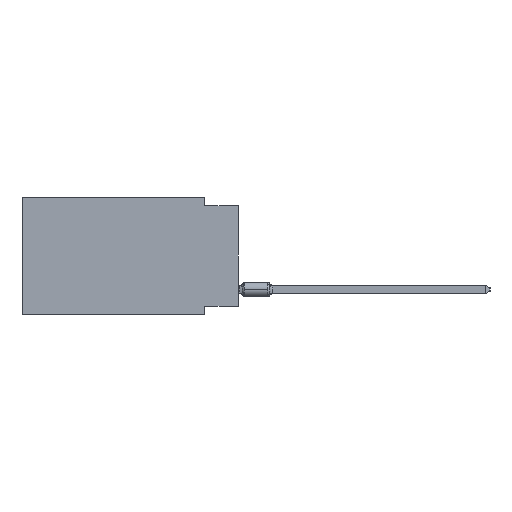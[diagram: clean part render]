
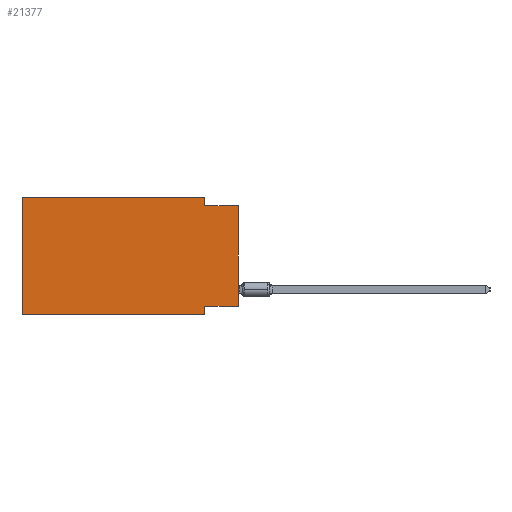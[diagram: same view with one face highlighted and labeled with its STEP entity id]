
A CAD part, left-side view. The second image highlights one B-rep face of the part: STEP entity #21377.
In plain terms, the highlighted planar face has unit normal (-1, 0, 0).
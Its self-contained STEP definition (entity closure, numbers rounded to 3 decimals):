
#441 = CARTESIAN_POINT ( 'NONE',  ( 0., 16.383, 0. ) ) ;
#513 = VECTOR ( 'NONE', #53998, 1000. ) ;
#1346 = DIRECTION ( 'NONE',  ( 0., 0., 1. ) ) ;
#3556 = VERTEX_POINT ( 'NONE', #6404 ) ;
#6296 = CARTESIAN_POINT ( 'NONE',  ( 0., 0., -0.635 ) ) ;
#6312 = CARTESIAN_POINT ( 'NONE',  ( 0., 0., -8.255 ) ) ;
#6404 = CARTESIAN_POINT ( 'NONE',  ( 0., 2.54, -8.89 ) ) ;
#7161 = VERTEX_POINT ( 'NONE', #33942 ) ;
#10131 = VECTOR ( 'NONE', #59134, 1000. ) ;
#10188 = VERTEX_POINT ( 'NONE', #39643 ) ;
#10349 = VERTEX_POINT ( 'NONE', #6312 ) ;
#10677 = VERTEX_POINT ( 'NONE', #50467 ) ;
#10801 = EDGE_CURVE ( 'NONE', #16293, #7161, #24238, .T. ) ;
#11159 = VECTOR ( 'NONE', #21275, 1000. ) ;
#12512 = DIRECTION ( 'NONE',  ( 0., 0., -1. ) ) ;
#13230 = VECTOR ( 'NONE', #26072, 1000. ) ;
#15696 = ORIENTED_EDGE ( 'NONE', *, *, #10801, .F. ) ;
#16110 = CARTESIAN_POINT ( 'NONE',  ( 0., 16.383, -8.89 ) ) ;
#16293 = VERTEX_POINT ( 'NONE', #16110 ) ;
#17406 = LINE ( 'NONE', #26827, #10131 ) ;
#18554 = EDGE_CURVE ( 'NONE', #10188, #3556, #17406, .T. ) ;
#20236 = VECTOR ( 'NONE', #42639, 1000. ) ;
#20433 = EDGE_LOOP ( 'NONE', ( #47919, #23058, #58850, #33932, #15696, #43660, #39591, #58017 ) ) ;
#20723 = EDGE_CURVE ( 'NONE', #10677, #45856, #34618, .T. ) ;
#21275 = DIRECTION ( 'NONE',  ( 0., -1., 0. ) ) ;
#21377 = ADVANCED_FACE ( 'NONE', ( #50583 ), #44787, .F. ) ;
#22853 = LINE ( 'NONE', #42329, #20236 ) ;
#23058 = ORIENTED_EDGE ( 'NONE', *, *, #20723, .F. ) ;
#23073 = VERTEX_POINT ( 'NONE', #57679 ) ;
#23483 = LINE ( 'NONE', #32929, #52231 ) ;
#23773 = EDGE_CURVE ( 'NONE', #10349, #10188, #28922, .T. ) ;
#24238 = LINE ( 'NONE', #441, #34769 ) ;
#25846 = EDGE_CURVE ( 'NONE', #10349, #45856, #22853, .T. ) ;
#26072 = DIRECTION ( 'NONE',  ( 0., -1., 0. ) ) ;
#26495 = CARTESIAN_POINT ( 'NONE',  ( 0., 16.383, 0. ) ) ;
#26827 = CARTESIAN_POINT ( 'NONE',  ( 0., 2.54, -8.89 ) ) ;
#27199 = EDGE_CURVE ( 'NONE', #16293, #3556, #34069, .T. ) ;
#28922 = LINE ( 'NONE', #42333, #38693 ) ;
#29515 = EDGE_CURVE ( 'NONE', #7161, #23073, #49119, .T. ) ;
#29878 = AXIS2_PLACEMENT_3D ( 'NONE', #26495, #40210, #12512 ) ;
#32929 = CARTESIAN_POINT ( 'NONE',  ( 0., 2.54, 0. ) ) ;
#33210 = DIRECTION ( 'NONE',  ( 0., 0., -1. ) ) ;
#33932 = ORIENTED_EDGE ( 'NONE', *, *, #29515, .F. ) ;
#33942 = CARTESIAN_POINT ( 'NONE',  ( 0., 16.383, 0. ) ) ;
#34069 = LINE ( 'NONE', #58132, #11159 ) ;
#34618 = LINE ( 'NONE', #34931, #13230 ) ;
#34769 = VECTOR ( 'NONE', #1346, 1000. ) ;
#34931 = CARTESIAN_POINT ( 'NONE',  ( 0., 0., -0.635 ) ) ;
#37191 = EDGE_CURVE ( 'NONE', #23073, #10677, #23483, .T. ) ;
#38058 = DIRECTION ( 'NONE',  ( 0., 1., 0. ) ) ;
#38693 = VECTOR ( 'NONE', #38058, 1000. ) ;
#39591 = ORIENTED_EDGE ( 'NONE', *, *, #18554, .F. ) ;
#39643 = CARTESIAN_POINT ( 'NONE',  ( 0., 2.54, -8.255 ) ) ;
#40210 = DIRECTION ( 'NONE',  ( 1., 0., 0. ) ) ;
#42329 = CARTESIAN_POINT ( 'NONE',  ( 0., 0., 0. ) ) ;
#42333 = CARTESIAN_POINT ( 'NONE',  ( 0., 0., -8.255 ) ) ;
#42639 = DIRECTION ( 'NONE',  ( 0., 0., 1. ) ) ;
#43660 = ORIENTED_EDGE ( 'NONE', *, *, #27199, .T. ) ;
#44251 = CARTESIAN_POINT ( 'NONE',  ( 0., 16.383, 0. ) ) ;
#44787 = PLANE ( 'NONE',  #29878 ) ;
#45856 = VERTEX_POINT ( 'NONE', #6296 ) ;
#47919 = ORIENTED_EDGE ( 'NONE', *, *, #25846, .T. ) ;
#49119 = LINE ( 'NONE', #44251, #513 ) ;
#50467 = CARTESIAN_POINT ( 'NONE',  ( 0., 2.54, -0.635 ) ) ;
#50583 = FACE_OUTER_BOUND ( 'NONE', #20433, .T. ) ;
#52231 = VECTOR ( 'NONE', #33210, 1000. ) ;
#53998 = DIRECTION ( 'NONE',  ( 0., -1., 0. ) ) ;
#57679 = CARTESIAN_POINT ( 'NONE',  ( 0., 2.54, 0. ) ) ;
#58017 = ORIENTED_EDGE ( 'NONE', *, *, #23773, .F. ) ;
#58132 = CARTESIAN_POINT ( 'NONE',  ( 0., 16.383, -8.89 ) ) ;
#58850 = ORIENTED_EDGE ( 'NONE', *, *, #37191, .F. ) ;
#59134 = DIRECTION ( 'NONE',  ( 0., 0., -1. ) ) ;
